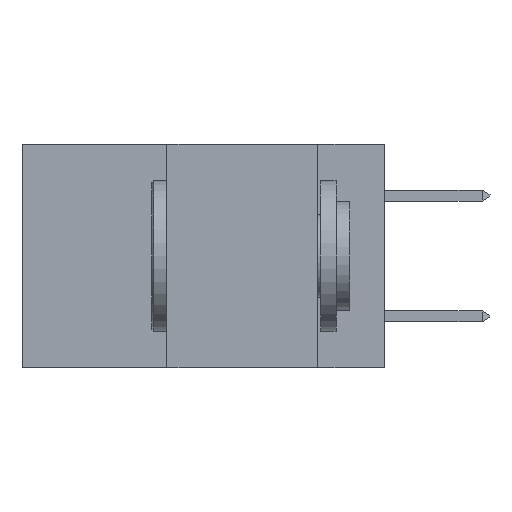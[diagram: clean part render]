
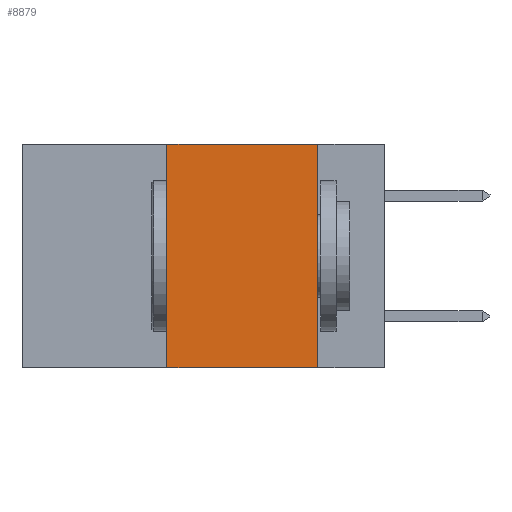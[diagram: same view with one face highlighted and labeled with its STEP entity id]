
A CAD part, left-side view. The second image highlights one B-rep face of the part: STEP entity #8879.
In plain terms, the highlighted planar face has unit normal (-1, 0, 0).
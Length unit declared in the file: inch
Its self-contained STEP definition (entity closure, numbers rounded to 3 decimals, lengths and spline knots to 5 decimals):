
#117 = CARTESIAN_POINT ( 'NONE',  ( 0., 0.36, 0. ) ) ;
#241 = CARTESIAN_POINT ( 'NONE',  ( 0., 0.6, -0.37 ) ) ;
#419 = EDGE_CURVE ( 'NONE', #7036, #10263, #3131, .T. ) ;
#634 = AXIS2_PLACEMENT_3D ( 'NONE', #21677, #16326, #5471 ) ;
#1354 = EDGE_CURVE ( 'NONE', #10263, #12677, #16744, .T. ) ;
#1752 = ORIENTED_EDGE ( 'NONE', *, *, #1354, .F. ) ;
#3131 = LINE ( 'NONE', #16438, #21816 ) ;
#3206 = CARTESIAN_POINT ( 'NONE',  ( 0., 0.11, -0.37 ) ) ;
#3427 = CARTESIAN_POINT ( 'NONE',  ( 0., 0.11, 0. ) ) ;
#3644 = PLANE ( 'NONE',  #634 ) ;
#4605 = VERTEX_POINT ( 'NONE', #5371 ) ;
#5371 = CARTESIAN_POINT ( 'NONE',  ( 0., 0.36, -0.37 ) ) ;
#5471 = DIRECTION ( 'NONE',  ( 0., 0., -1. ) ) ;
#7036 = VERTEX_POINT ( 'NONE', #117 ) ;
#7144 = VECTOR ( 'NONE', #13588, 39.37008 ) ;
#8879 = ADVANCED_FACE ( 'NONE', ( #22868 ), #3644, .F. ) ;
#9488 = ORIENTED_EDGE ( 'NONE', *, *, #11777, .T. ) ;
#9771 = DIRECTION ( 'NONE',  ( 0., -1., 0. ) ) ;
#10263 = VERTEX_POINT ( 'NONE', #3427 ) ;
#11777 = EDGE_CURVE ( 'NONE', #4605, #12677, #17389, .T. ) ;
#12039 = VECTOR ( 'NONE', #14764, 39.37008 ) ;
#12677 = VERTEX_POINT ( 'NONE', #3206 ) ;
#13235 = EDGE_LOOP ( 'NONE', ( #1752, #16805, #22722, #9488 ) ) ;
#13345 = LINE ( 'NONE', #13857, #22380 ) ;
#13588 = DIRECTION ( 'NONE',  ( 0., 0., -1. ) ) ;
#13645 = CARTESIAN_POINT ( 'NONE',  ( 0., 0.11, 0. ) ) ;
#13857 = CARTESIAN_POINT ( 'NONE',  ( 0., 0.36, 0. ) ) ;
#14764 = DIRECTION ( 'NONE',  ( 0., -1., 0. ) ) ;
#15666 = DIRECTION ( 'NONE',  ( 0., 0., 1. ) ) ;
#16326 = DIRECTION ( 'NONE',  ( 1., 0., 0. ) ) ;
#16438 = CARTESIAN_POINT ( 'NONE',  ( 0., 0.6, 0. ) ) ;
#16744 = LINE ( 'NONE', #13645, #7144 ) ;
#16805 = ORIENTED_EDGE ( 'NONE', *, *, #419, .F. ) ;
#17389 = LINE ( 'NONE', #241, #12039 ) ;
#20988 = EDGE_CURVE ( 'NONE', #4605, #7036, #13345, .T. ) ;
#21677 = CARTESIAN_POINT ( 'NONE',  ( 0., 0.6, 0. ) ) ;
#21816 = VECTOR ( 'NONE', #9771, 39.37008 ) ;
#22380 = VECTOR ( 'NONE', #15666, 39.37008 ) ;
#22722 = ORIENTED_EDGE ( 'NONE', *, *, #20988, .F. ) ;
#22868 = FACE_OUTER_BOUND ( 'NONE', #13235, .T. ) ;
